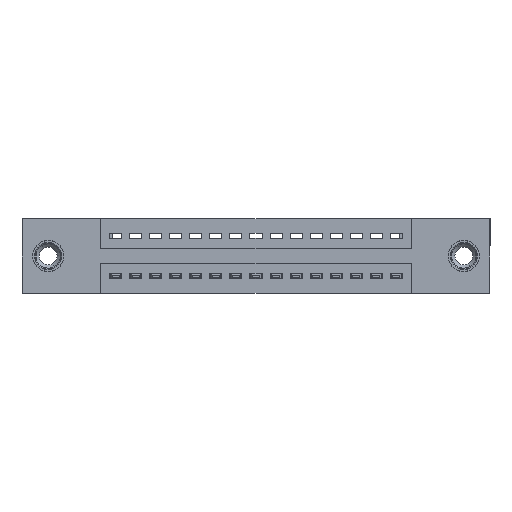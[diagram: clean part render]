
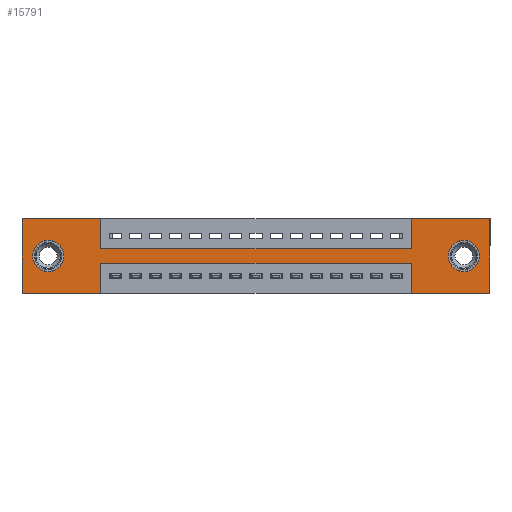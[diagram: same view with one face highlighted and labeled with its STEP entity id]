
A CAD part, front view. The second image highlights one B-rep face of the part: STEP entity #15791.
In plain terms, the highlighted planar face has unit normal (0, -1, 0).
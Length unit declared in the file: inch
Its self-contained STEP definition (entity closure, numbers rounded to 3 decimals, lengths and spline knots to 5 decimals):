
#135 = EDGE_CURVE ( 'NONE', #15394, #7318, #18575, .T. ) ;
#167 = CIRCLE ( 'NONE', #16746, 0.078 ) ;
#219 = AXIS2_PLACEMENT_3D ( 'NONE', #19003, #11886, #2884 ) ;
#304 = DIRECTION ( 'NONE',  ( 0., 0., -1. ) ) ;
#321 = VECTOR ( 'NONE', #12373, 39.37008 ) ;
#330 = CARTESIAN_POINT ( 'NONE',  ( 2.335, 0., 0. ) ) ;
#356 = ORIENTED_EDGE ( 'NONE', *, *, #14524, .F. ) ;
#606 = ORIENTED_EDGE ( 'NONE', *, *, #16276, .F. ) ;
#841 = EDGE_CURVE ( 'NONE', #7318, #15394, #167, .T. ) ;
#1645 = CARTESIAN_POINT ( 'NONE',  ( 0., 0., 0. ) ) ;
#1696 = CARTESIAN_POINT ( 'NONE',  ( 1.9425, 0., -0.15 ) ) ;
#1797 = CARTESIAN_POINT ( 'NONE',  ( 0., 0., -0.37 ) ) ;
#1807 = LINE ( 'NONE', #11117, #11216 ) ;
#1848 = VERTEX_POINT ( 'NONE', #4066 ) ;
#1918 = ORIENTED_EDGE ( 'NONE', *, *, #10334, .F. ) ;
#2004 = ORIENTED_EDGE ( 'NONE', *, *, #16952, .F. ) ;
#2246 = VERTEX_POINT ( 'NONE', #14873 ) ;
#2255 = VERTEX_POINT ( 'NONE', #13586 ) ;
#2285 = CARTESIAN_POINT ( 'NONE',  ( 0., 0., 0. ) ) ;
#2377 = CARTESIAN_POINT ( 'NONE',  ( 0.3925, 0., -0.37 ) ) ;
#2647 = DIRECTION ( 'NONE',  ( 0., 0., 1. ) ) ;
#2659 = VECTOR ( 'NONE', #9554, 39.37008 ) ;
#2696 = EDGE_CURVE ( 'NONE', #6742, #18908, #3403, .T. ) ;
#2884 = DIRECTION ( 'NONE',  ( 0., 0., 1. ) ) ;
#3122 = ORIENTED_EDGE ( 'NONE', *, *, #12000, .F. ) ;
#3156 = VERTEX_POINT ( 'NONE', #17694 ) ;
#3361 = CARTESIAN_POINT ( 'NONE',  ( 2.205, 0., -0.185 ) ) ;
#3393 = AXIS2_PLACEMENT_3D ( 'NONE', #13894, #3562, #9917 ) ;
#3403 = LINE ( 'NONE', #7031, #6949 ) ;
#3413 = VERTEX_POINT ( 'NONE', #3801 ) ;
#3527 = ORIENTED_EDGE ( 'NONE', *, *, #841, .T. ) ;
#3562 = DIRECTION ( 'NONE',  ( 0., 1., 0. ) ) ;
#3640 = VERTEX_POINT ( 'NONE', #10684 ) ;
#3801 = CARTESIAN_POINT ( 'NONE',  ( 2.335, 0., 0. ) ) ;
#3809 = ORIENTED_EDGE ( 'NONE', *, *, #19264, .F. ) ;
#4066 = CARTESIAN_POINT ( 'NONE',  ( 1.9425, 0., 0. ) ) ;
#4206 = CARTESIAN_POINT ( 'NONE',  ( 0.13, 0., -0.263 ) ) ;
#4703 = CARTESIAN_POINT ( 'NONE',  ( 2.205, 0., -0.107 ) ) ;
#4855 = VECTOR ( 'NONE', #18230, 39.37008 ) ;
#4935 = CARTESIAN_POINT ( 'NONE',  ( 0.3925, 0., -0.22 ) ) ;
#5369 = DIRECTION ( 'NONE',  ( 1., 0., 0. ) ) ;
#5981 = EDGE_LOOP ( 'NONE', ( #8117, #10108 ) ) ;
#6144 = CIRCLE ( 'NONE', #219, 0.078 ) ;
#6577 = CARTESIAN_POINT ( 'NONE',  ( 0.3925, 0., -0.15 ) ) ;
#6718 = LINE ( 'NONE', #1797, #321 ) ;
#6742 = VERTEX_POINT ( 'NONE', #13017 ) ;
#6915 = ORIENTED_EDGE ( 'NONE', *, *, #10957, .F. ) ;
#6949 = VECTOR ( 'NONE', #8446, 39.37008 ) ;
#7031 = CARTESIAN_POINT ( 'NONE',  ( 0.3925, 0., -0.37 ) ) ;
#7318 = VERTEX_POINT ( 'NONE', #17110 ) ;
#7462 = VECTOR ( 'NONE', #5369, 39.37008 ) ;
#7728 = CARTESIAN_POINT ( 'NONE',  ( 0., 0., -0.37 ) ) ;
#7731 = DIRECTION ( 'NONE',  ( 0., 0., -1. ) ) ;
#7968 = ORIENTED_EDGE ( 'NONE', *, *, #8476, .F. ) ;
#8117 = ORIENTED_EDGE ( 'NONE', *, *, #14091, .T. ) ;
#8155 = DIRECTION ( 'NONE',  ( 1., 0., 0. ) ) ;
#8316 = PLANE ( 'NONE',  #18552 ) ;
#8446 = DIRECTION ( 'NONE',  ( 0., 0., -1. ) ) ;
#8476 = EDGE_CURVE ( 'NONE', #16633, #2255, #16376, .T. ) ;
#8883 = VERTEX_POINT ( 'NONE', #13173 ) ;
#9005 = LINE ( 'NONE', #12153, #14872 ) ;
#9419 = VECTOR ( 'NONE', #9492, 39.37008 ) ;
#9491 = DIRECTION ( 'NONE',  ( 1., 0., 0. ) ) ;
#9492 = DIRECTION ( 'NONE',  ( -1., 0., 0. ) ) ;
#9554 = DIRECTION ( 'NONE',  ( 0., 0., 1. ) ) ;
#9626 = EDGE_CURVE ( 'NONE', #18908, #18701, #17046, .T. ) ;
#9829 = DIRECTION ( 'NONE',  ( 0., 0., -1. ) ) ;
#9902 = CARTESIAN_POINT ( 'NONE',  ( 0., 0., -0.37 ) ) ;
#9917 = DIRECTION ( 'NONE',  ( 0., 0., 1. ) ) ;
#10108 = ORIENTED_EDGE ( 'NONE', *, *, #12590, .T. ) ;
#10287 = EDGE_CURVE ( 'NONE', #3640, #15401, #13029, .T. ) ;
#10334 = EDGE_CURVE ( 'NONE', #15401, #1848, #11131, .T. ) ;
#10684 = CARTESIAN_POINT ( 'NONE',  ( 0.3925, 0., -0.15 ) ) ;
#10911 = ORIENTED_EDGE ( 'NONE', *, *, #135, .T. ) ;
#10956 = LINE ( 'NONE', #2285, #12598 ) ;
#10957 = EDGE_CURVE ( 'NONE', #18701, #16633, #11555, .T. ) ;
#11002 = CARTESIAN_POINT ( 'NONE',  ( 1.9425, 0., 0. ) ) ;
#11117 = CARTESIAN_POINT ( 'NONE',  ( 1.9425, 0., -0.37 ) ) ;
#11131 = LINE ( 'NONE', #11002, #2659 ) ;
#11216 = VECTOR ( 'NONE', #14248, 39.37008 ) ;
#11555 = LINE ( 'NONE', #11720, #16517 ) ;
#11720 = CARTESIAN_POINT ( 'NONE',  ( 0., 0., 0. ) ) ;
#11886 = DIRECTION ( 'NONE',  ( 0., 1., 0. ) ) ;
#12000 = EDGE_CURVE ( 'NONE', #3156, #6742, #17176, .T. ) ;
#12022 = DIRECTION ( 'NONE',  ( 0., 1., 0. ) ) ;
#12153 = CARTESIAN_POINT ( 'NONE',  ( 0.3925, 0., 0. ) ) ;
#12291 = DIRECTION ( 'NONE',  ( 0., 0., -1. ) ) ;
#12331 = ORIENTED_EDGE ( 'NONE', *, *, #10287, .F. ) ;
#12373 = DIRECTION ( 'NONE',  ( -1., 0., 0. ) ) ;
#12462 = VECTOR ( 'NONE', #7731, 39.37008 ) ;
#12590 = EDGE_CURVE ( 'NONE', #14748, #13666, #6144, .T. ) ;
#12598 = VECTOR ( 'NONE', #8155, 39.37008 ) ;
#12637 = FACE_BOUND ( 'NONE', #13524, .T. ) ;
#12760 = EDGE_LOOP ( 'NONE', ( #16998, #3122, #606, #15905, #356, #2004, #1918, #12331, #3809, #7968, #6915, #19347 ) ) ;
#12996 = DIRECTION ( 'NONE',  ( 0., -1., 0. ) ) ;
#13017 = CARTESIAN_POINT ( 'NONE',  ( 0.3925, 0., -0.22 ) ) ;
#13029 = LINE ( 'NONE', #6577, #16774 ) ;
#13173 = CARTESIAN_POINT ( 'NONE',  ( 1.9425, 0., -0.37 ) ) ;
#13524 = EDGE_LOOP ( 'NONE', ( #10911, #3527 ) ) ;
#13586 = CARTESIAN_POINT ( 'NONE',  ( 0.3925, 0., 0. ) ) ;
#13666 = VERTEX_POINT ( 'NONE', #15187 ) ;
#13705 = CARTESIAN_POINT ( 'NONE',  ( 0., 0., -0.37 ) ) ;
#13894 = CARTESIAN_POINT ( 'NONE',  ( 0.13, 0., -0.185 ) ) ;
#14091 = EDGE_CURVE ( 'NONE', #13666, #14748, #18610, .T. ) ;
#14097 = LINE ( 'NONE', #330, #12462 ) ;
#14248 = DIRECTION ( 'NONE',  ( 0., 0., 1. ) ) ;
#14524 = EDGE_CURVE ( 'NONE', #3413, #2246, #14097, .T. ) ;
#14748 = VERTEX_POINT ( 'NONE', #4206 ) ;
#14872 = VECTOR ( 'NONE', #12291, 39.37008 ) ;
#14873 = CARTESIAN_POINT ( 'NONE',  ( 2.335, 0., -0.37 ) ) ;
#15187 = CARTESIAN_POINT ( 'NONE',  ( 0.13, 0., -0.107 ) ) ;
#15394 = VERTEX_POINT ( 'NONE', #4703 ) ;
#15401 = VERTEX_POINT ( 'NONE', #1696 ) ;
#15791 = ADVANCED_FACE ( 'NONE', ( #12637, #17349, #16406 ), #8316, .T. ) ;
#15905 = ORIENTED_EDGE ( 'NONE', *, *, #17854, .F. ) ;
#16276 = EDGE_CURVE ( 'NONE', #8883, #3156, #1807, .T. ) ;
#16376 = LINE ( 'NONE', #16703, #7462 ) ;
#16406 = FACE_OUTER_BOUND ( 'NONE', #12760, .T. ) ;
#16517 = VECTOR ( 'NONE', #2647, 39.37008 ) ;
#16633 = VERTEX_POINT ( 'NONE', #1645 ) ;
#16703 = CARTESIAN_POINT ( 'NONE',  ( 0., 0., 0. ) ) ;
#16746 = AXIS2_PLACEMENT_3D ( 'NONE', #3361, #12022, #18017 ) ;
#16774 = VECTOR ( 'NONE', #9491, 39.37008 ) ;
#16952 = EDGE_CURVE ( 'NONE', #1848, #3413, #10956, .T. ) ;
#16998 = ORIENTED_EDGE ( 'NONE', *, *, #2696, .F. ) ;
#17046 = LINE ( 'NONE', #7728, #4855 ) ;
#17110 = CARTESIAN_POINT ( 'NONE',  ( 2.205, 0., -0.263 ) ) ;
#17176 = LINE ( 'NONE', #4935, #9419 ) ;
#17349 = FACE_BOUND ( 'NONE', #5981, .T. ) ;
#17694 = CARTESIAN_POINT ( 'NONE',  ( 1.9425, 0., -0.22 ) ) ;
#17854 = EDGE_CURVE ( 'NONE', #2246, #8883, #6718, .T. ) ;
#17877 = CARTESIAN_POINT ( 'NONE',  ( 2.205, 0., -0.185 ) ) ;
#18007 = DIRECTION ( 'NONE',  ( 0., 1., 0. ) ) ;
#18017 = DIRECTION ( 'NONE',  ( 0., 0., -1. ) ) ;
#18230 = DIRECTION ( 'NONE',  ( -1., 0., 0. ) ) ;
#18552 = AXIS2_PLACEMENT_3D ( 'NONE', #9902, #12996, #9829 ) ;
#18575 = CIRCLE ( 'NONE', #18773, 0.078 ) ;
#18610 = CIRCLE ( 'NONE', #3393, 0.078 ) ;
#18701 = VERTEX_POINT ( 'NONE', #13705 ) ;
#18773 = AXIS2_PLACEMENT_3D ( 'NONE', #17877, #18007, #304 ) ;
#18908 = VERTEX_POINT ( 'NONE', #2377 ) ;
#19003 = CARTESIAN_POINT ( 'NONE',  ( 0.13, 0., -0.185 ) ) ;
#19264 = EDGE_CURVE ( 'NONE', #2255, #3640, #9005, .T. ) ;
#19347 = ORIENTED_EDGE ( 'NONE', *, *, #9626, .F. ) ;
